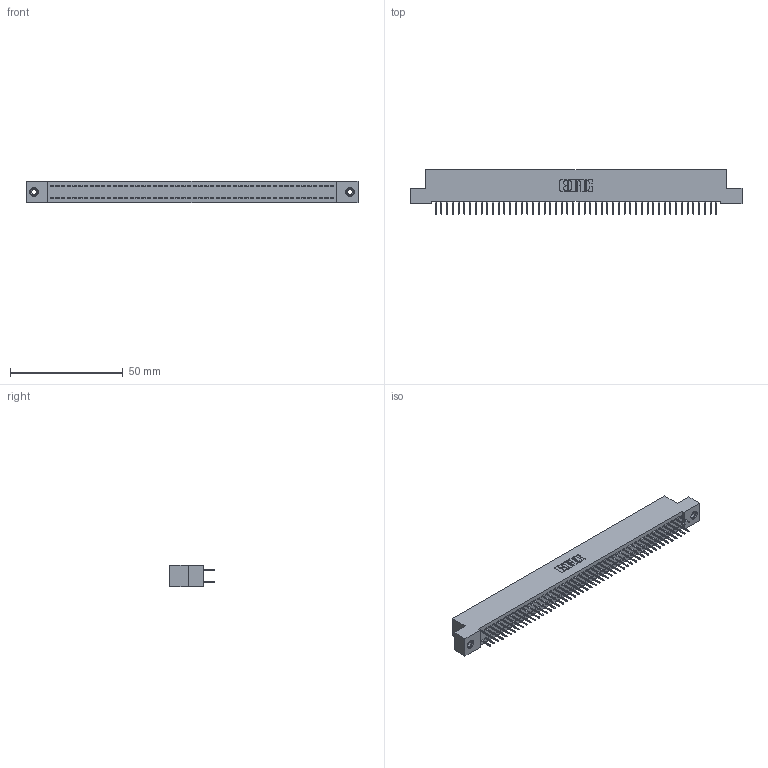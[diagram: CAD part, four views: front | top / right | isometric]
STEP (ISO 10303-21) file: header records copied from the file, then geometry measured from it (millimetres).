
FILE_DESCRIPTION (( 'STEP AP203' ), '1' );
FILE_NAME ('392-100-524-208.STEP', '2019-10-09T20:49:27', ( '' ), ( '' ), 'SwSTEP 2.0', 'SolidWorks 2016', '' );
FILE_SCHEMA (( 'CONFIG_CONTROL_DESIGN' ));
Length unit declared in the file: inch
Products named in the file (4): 342 Part_TI; 345-292-001_345-293-124; 345-250-001_345-250-003-102; 392-100-524-208
Assembly tree (103 placements, depth 2):
  392-100-524-208
    342 Part_TI
    345-292-001_345-293-124  x100
    345-250-001_345-250-003-102  x2
Bounding box: 147.32 x 19.69 x 9.4 mm (x, y, z)
Volume: 13117.5 mm3; surface area: 21165.8 mm2
Topology: 103 solids, 103 shells, 5770 faces, 16335 edges, 10482 vertices
Faces by surface type: plane 4298, cylinder 1456, cone 12, torus 4
Entity records: 32260 total; most frequent: CARTESIAN_POINT 5317, ORIENTED_EDGE 5246, DIRECTION 4561, EDGE_CURVE 2623, LINE 2479, VECTOR 2479, VERTEX_POINT 1740, AXIS2_PLACEMENT_3D 1041
